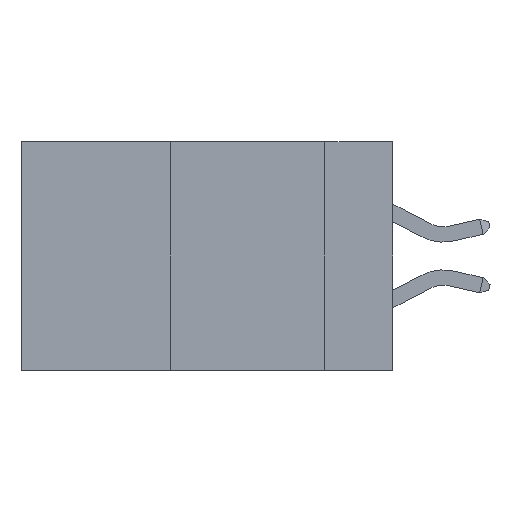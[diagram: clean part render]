
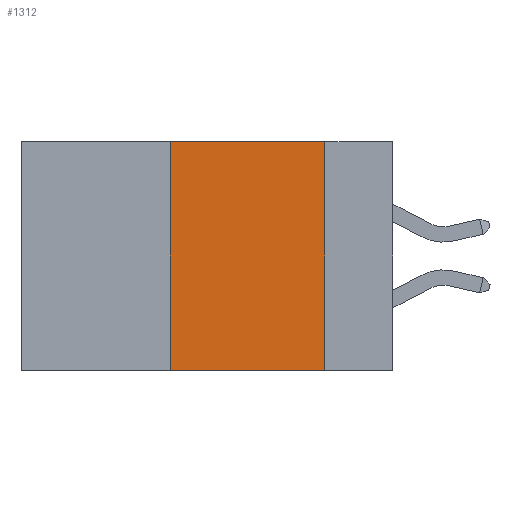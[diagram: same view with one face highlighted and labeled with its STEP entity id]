
A CAD part, left-side view. The second image highlights one B-rep face of the part: STEP entity #1312.
In plain terms, the highlighted planar face has unit normal (-1, 0, 0).
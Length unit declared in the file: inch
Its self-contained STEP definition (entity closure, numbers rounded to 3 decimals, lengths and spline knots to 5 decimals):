
#169 = CARTESIAN_POINT ( 'NONE',  ( 0., 0.36, -0.37 ) ) ;
#390 = EDGE_LOOP ( 'NONE', ( #12704, #22672, #9018, #23222 ) ) ;
#1312 = ADVANCED_FACE ( 'NONE', ( #5870 ), #16809, .F. ) ;
#1753 = DIRECTION ( 'NONE',  ( 0., 0., -1. ) ) ;
#3982 = CARTESIAN_POINT ( 'NONE',  ( 0., 0.6, 0. ) ) ;
#5870 = FACE_OUTER_BOUND ( 'NONE', #390, .T. ) ;
#6299 = CARTESIAN_POINT ( 'NONE',  ( 0., 0.11, -0.37 ) ) ;
#6683 = EDGE_CURVE ( 'NONE', #12897, #12795, #19174, .T. ) ;
#6740 = VECTOR ( 'NONE', #20069, 39.37008 ) ;
#7354 = CARTESIAN_POINT ( 'NONE',  ( 0., 0.11, 0. ) ) ;
#7777 = DIRECTION ( 'NONE',  ( 0., -1., 0. ) ) ;
#7810 = VECTOR ( 'NONE', #1753, 39.37008 ) ;
#7877 = EDGE_CURVE ( 'NONE', #8414, #12197, #11337, .T. ) ;
#8290 = LINE ( 'NONE', #16261, #21418 ) ;
#8414 = VERTEX_POINT ( 'NONE', #169 ) ;
#9018 = ORIENTED_EDGE ( 'NONE', *, *, #21358, .F. ) ;
#9458 = CARTESIAN_POINT ( 'NONE',  ( 0., 0.36, 0. ) ) ;
#9666 = DIRECTION ( 'NONE',  ( 1., 0., 0. ) ) ;
#11337 = LINE ( 'NONE', #13156, #20196 ) ;
#12197 = VERTEX_POINT ( 'NONE', #6299 ) ;
#12628 = CARTESIAN_POINT ( 'NONE',  ( 0., 0.11, 0. ) ) ;
#12704 = ORIENTED_EDGE ( 'NONE', *, *, #15291, .F. ) ;
#12795 = VERTEX_POINT ( 'NONE', #7354 ) ;
#12897 = VERTEX_POINT ( 'NONE', #9458 ) ;
#13156 = CARTESIAN_POINT ( 'NONE',  ( 0., 0.6, -0.37 ) ) ;
#14494 = DIRECTION ( 'NONE',  ( 0., 0., 1. ) ) ;
#15291 = EDGE_CURVE ( 'NONE', #12795, #12197, #21495, .T. ) ;
#16261 = CARTESIAN_POINT ( 'NONE',  ( 0., 0.36, 0. ) ) ;
#16809 = PLANE ( 'NONE',  #22449 ) ;
#19174 = LINE ( 'NONE', #3982, #6740 ) ;
#20069 = DIRECTION ( 'NONE',  ( 0., -1., 0. ) ) ;
#20196 = VECTOR ( 'NONE', #7777, 39.37008 ) ;
#20323 = CARTESIAN_POINT ( 'NONE',  ( 0., 0.6, 0. ) ) ;
#21358 = EDGE_CURVE ( 'NONE', #8414, #12897, #8290, .T. ) ;
#21418 = VECTOR ( 'NONE', #14494, 39.37008 ) ;
#21495 = LINE ( 'NONE', #12628, #7810 ) ;
#22139 = DIRECTION ( 'NONE',  ( 0., 0., -1. ) ) ;
#22449 = AXIS2_PLACEMENT_3D ( 'NONE', #20323, #9666, #22139 ) ;
#22672 = ORIENTED_EDGE ( 'NONE', *, *, #6683, .F. ) ;
#23222 = ORIENTED_EDGE ( 'NONE', *, *, #7877, .T. ) ;
